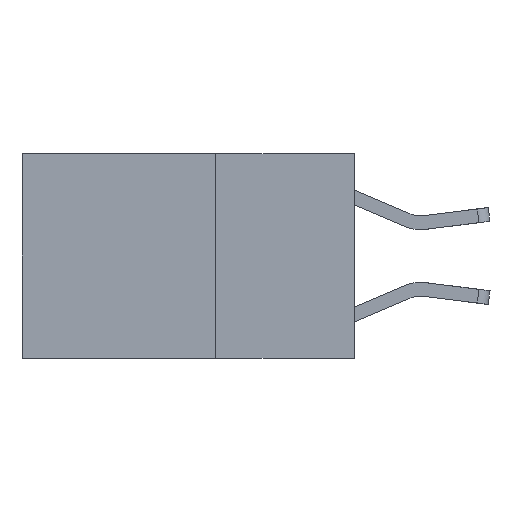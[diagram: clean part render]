
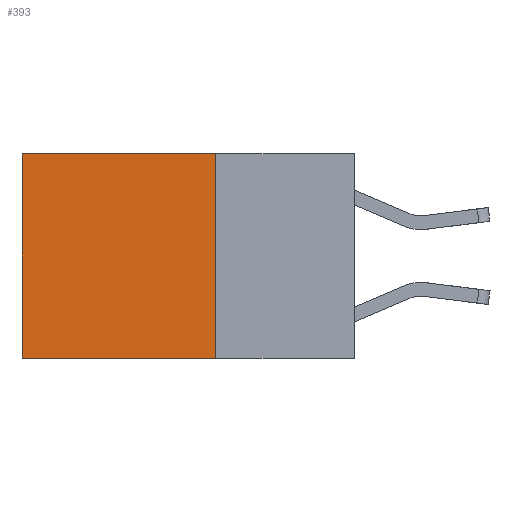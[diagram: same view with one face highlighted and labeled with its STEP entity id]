
A CAD part, left-side view. The second image highlights one B-rep face of the part: STEP entity #393.
In plain terms, the highlighted planar face has unit normal (-1, 0, 0).
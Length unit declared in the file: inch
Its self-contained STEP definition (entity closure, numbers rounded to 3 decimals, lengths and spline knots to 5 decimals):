
#162 = ORIENTED_EDGE ( 'NONE', *, *, #5128, .T. ) ;
#393 = ADVANCED_FACE ( 'NONE', ( #8512 ), #1031, .F. ) ;
#1031 = PLANE ( 'NONE',  #4034 ) ;
#1723 = LINE ( 'NONE', #1873, #5149 ) ;
#1873 = CARTESIAN_POINT ( 'NONE',  ( 0.2625, 0.25, 0. ) ) ;
#1900 = CARTESIAN_POINT ( 'NONE',  ( 0.2625, 0.25, -0.37 ) ) ;
#2082 = DIRECTION ( 'NONE',  ( 0., 0., -1. ) ) ;
#2095 = VERTEX_POINT ( 'NONE', #5969 ) ;
#2320 = VERTEX_POINT ( 'NONE', #2955 ) ;
#2459 = LINE ( 'NONE', #3198, #4077 ) ;
#2635 = EDGE_CURVE ( 'NONE', #4588, #6751, #6748, .T. ) ;
#2763 = ORIENTED_EDGE ( 'NONE', *, *, #4748, .F. ) ;
#2800 = CARTESIAN_POINT ( 'NONE',  ( 0.2625, 0.25, 0. ) ) ;
#2955 = CARTESIAN_POINT ( 'NONE',  ( 0.2625, 0.6, 0. ) ) ;
#3198 = CARTESIAN_POINT ( 'NONE',  ( 0.2625, 0.6, 0. ) ) ;
#3944 = DIRECTION ( 'NONE',  ( 0., 1., 0. ) ) ;
#4034 = AXIS2_PLACEMENT_3D ( 'NONE', #8106, #6604, #7170 ) ;
#4077 = VECTOR ( 'NONE', #7333, 39.37008 ) ;
#4569 = EDGE_CURVE ( 'NONE', #2095, #2320, #1723, .T. ) ;
#4588 = VERTEX_POINT ( 'NONE', #1900 ) ;
#4748 = EDGE_CURVE ( 'NONE', #2095, #4588, #5261, .T. ) ;
#4976 = EDGE_LOOP ( 'NONE', ( #162, #6245, #2763, #8199 ) ) ;
#5128 = EDGE_CURVE ( 'NONE', #2320, #6751, #2459, .T. ) ;
#5149 = VECTOR ( 'NONE', #3944, 39.37008 ) ;
#5261 = LINE ( 'NONE', #2800, #8604 ) ;
#5969 = CARTESIAN_POINT ( 'NONE',  ( 0.2625, 0.25, 0. ) ) ;
#6245 = ORIENTED_EDGE ( 'NONE', *, *, #2635, .F. ) ;
#6356 = CARTESIAN_POINT ( 'NONE',  ( 0.2625, 0.6, -0.37 ) ) ;
#6604 = DIRECTION ( 'NONE',  ( 1., 0., 0. ) ) ;
#6748 = LINE ( 'NONE', #7018, #8259 ) ;
#6751 = VERTEX_POINT ( 'NONE', #6356 ) ;
#6963 = DIRECTION ( 'NONE',  ( 0., 1., 0. ) ) ;
#7018 = CARTESIAN_POINT ( 'NONE',  ( 0.2625, 0.25, -0.37 ) ) ;
#7170 = DIRECTION ( 'NONE',  ( 0., 0., -1. ) ) ;
#7333 = DIRECTION ( 'NONE',  ( 0., 0., -1. ) ) ;
#8106 = CARTESIAN_POINT ( 'NONE',  ( 0.2625, 0.25, 0. ) ) ;
#8199 = ORIENTED_EDGE ( 'NONE', *, *, #4569, .T. ) ;
#8259 = VECTOR ( 'NONE', #6963, 39.37008 ) ;
#8512 = FACE_OUTER_BOUND ( 'NONE', #4976, .T. ) ;
#8604 = VECTOR ( 'NONE', #2082, 39.37008 ) ;
